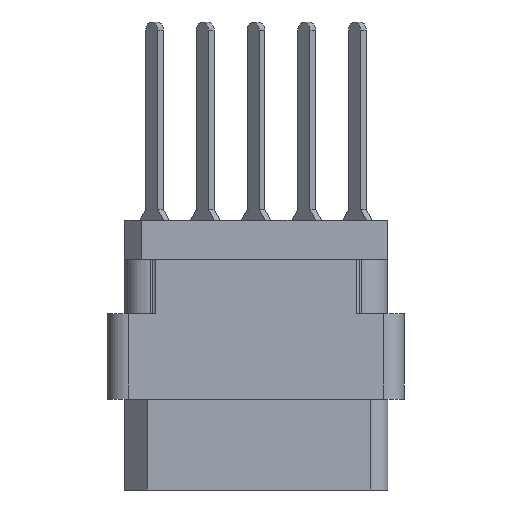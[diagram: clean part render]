
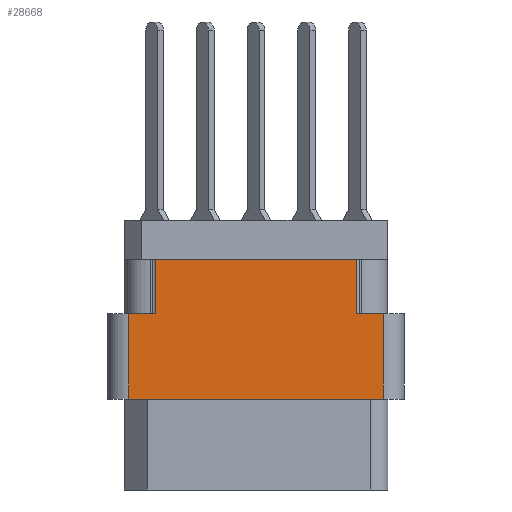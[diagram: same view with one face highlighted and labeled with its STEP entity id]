
A CAD part, left-side view. The second image highlights one B-rep face of the part: STEP entity #28668.
In plain terms, the highlighted planar face has unit normal (-1, 0, 0).
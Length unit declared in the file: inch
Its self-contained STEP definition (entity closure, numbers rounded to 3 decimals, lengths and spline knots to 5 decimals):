
#728 = CARTESIAN_POINT ( 'NONE',  ( -1., -0.376, -0.277 ) ) ;
#792 = LINE ( 'NONE', #17504, #22685 ) ;
#1238 = ORIENTED_EDGE ( 'NONE', *, *, #32346, .F. ) ;
#1358 = VECTOR ( 'NONE', #21945, 39.37008 ) ;
#1359 = EDGE_CURVE ( 'NONE', #29401, #2110, #792, .T. ) ;
#1814 = VECTOR ( 'NONE', #14646, 39.37008 ) ;
#2110 = VERTEX_POINT ( 'NONE', #22206 ) ;
#2185 = CARTESIAN_POINT ( 'NONE',  ( -1., -0.376, -0.529 ) ) ;
#2782 = CARTESIAN_POINT ( 'NONE',  ( -1., -0.376, -0.798 ) ) ;
#3081 = LINE ( 'NONE', #23075, #1814 ) ;
#3277 = DIRECTION ( 'NONE',  ( 0., -1., 0. ) ) ;
#3283 = CARTESIAN_POINT ( 'NONE',  ( -1., 0.376, -0.529 ) ) ;
#3299 = LINE ( 'NONE', #28642, #33651 ) ;
#4093 = DIRECTION ( 'NONE',  ( 0., -1., 0. ) ) ;
#4185 = VERTEX_POINT ( 'NONE', #6062 ) ;
#4687 = VERTEX_POINT ( 'NONE', #3283 ) ;
#4744 = VERTEX_POINT ( 'NONE', #35424 ) ;
#6062 = CARTESIAN_POINT ( 'NONE',  ( -1., -0.376, -0.529 ) ) ;
#6302 = EDGE_CURVE ( 'NONE', #4185, #4687, #10773, .T. ) ;
#7839 = VERTEX_POINT ( 'NONE', #728 ) ;
#8402 = CARTESIAN_POINT ( 'NONE',  ( -1., 0.438, -0.277 ) ) ;
#9349 = CARTESIAN_POINT ( 'NONE',  ( -1., 0.296, -0.277 ) ) ;
#9473 = VERTEX_POINT ( 'NONE', #10988 ) ;
#9908 = EDGE_CURVE ( 'NONE', #4744, #2110, #19010, .T. ) ;
#10062 = ORIENTED_EDGE ( 'NONE', *, *, #17559, .T. ) ;
#10773 = LINE ( 'NONE', #2185, #28179 ) ;
#10988 = CARTESIAN_POINT ( 'NONE',  ( -1., 0.376, -0.277 ) ) ;
#12277 = ORIENTED_EDGE ( 'NONE', *, *, #29274, .F. ) ;
#13438 = DIRECTION ( 'NONE',  ( 0., 0., 1. ) ) ;
#13970 = EDGE_LOOP ( 'NONE', ( #18472, #18614, #10062, #1238, #22683, #14006, #21763, #12277 ) ) ;
#14006 = ORIENTED_EDGE ( 'NONE', *, *, #1359, .F. ) ;
#14646 = DIRECTION ( 'NONE',  ( 0., 0., 1. ) ) ;
#14798 = DIRECTION ( 'NONE',  ( 0., 0., 1. ) ) ;
#15118 = VECTOR ( 'NONE', #3277, 39.37008 ) ;
#17504 = CARTESIAN_POINT ( 'NONE',  ( -1., 0.438, -0.117 ) ) ;
#17559 = EDGE_CURVE ( 'NONE', #4185, #7839, #3299, .T. ) ;
#18472 = ORIENTED_EDGE ( 'NONE', *, *, #19358, .F. ) ;
#18614 = ORIENTED_EDGE ( 'NONE', *, *, #6302, .F. ) ;
#19010 = LINE ( 'NONE', #33187, #1358 ) ;
#19358 = EDGE_CURVE ( 'NONE', #4687, #9473, #34122, .T. ) ;
#19970 = LINE ( 'NONE', #31565, #28435 ) ;
#21763 = ORIENTED_EDGE ( 'NONE', *, *, #24199, .F. ) ;
#21869 = PLANE ( 'NONE',  #32111 ) ;
#21945 = DIRECTION ( 'NONE',  ( 0., 0., 1. ) ) ;
#22206 = CARTESIAN_POINT ( 'NONE',  ( -1., -0.296, -0.117 ) ) ;
#22683 = ORIENTED_EDGE ( 'NONE', *, *, #9908, .T. ) ;
#22685 = VECTOR ( 'NONE', #4093, 39.37008 ) ;
#23075 = CARTESIAN_POINT ( 'NONE',  ( -1., 0.296, -0.277 ) ) ;
#24199 = EDGE_CURVE ( 'NONE', #30177, #29401, #3081, .T. ) ;
#25002 = FACE_OUTER_BOUND ( 'NONE', #13970, .T. ) ;
#25105 = DIRECTION ( 'NONE',  ( 0., 1., 0. ) ) ;
#28179 = VECTOR ( 'NONE', #25105, 39.37008 ) ;
#28246 = LINE ( 'NONE', #8402, #15118 ) ;
#28435 = VECTOR ( 'NONE', #31190, 39.37008 ) ;
#28642 = CARTESIAN_POINT ( 'NONE',  ( -1., -0.376, -0.798 ) ) ;
#28668 = ADVANCED_FACE ( 'NONE', ( #25002 ), #21869, .T. ) ;
#29166 = CARTESIAN_POINT ( 'NONE',  ( -1., 0.296, -0.117 ) ) ;
#29274 = EDGE_CURVE ( 'NONE', #9473, #30177, #28246, .T. ) ;
#29401 = VERTEX_POINT ( 'NONE', #29166 ) ;
#30177 = VERTEX_POINT ( 'NONE', #9349 ) ;
#31014 = CARTESIAN_POINT ( 'NONE',  ( -1., 0.376, -0.798 ) ) ;
#31190 = DIRECTION ( 'NONE',  ( 0., -1., 0. ) ) ;
#31214 = DIRECTION ( 'NONE',  ( 0., 0., 1. ) ) ;
#31565 = CARTESIAN_POINT ( 'NONE',  ( -1., -0.296, -0.277 ) ) ;
#32111 = AXIS2_PLACEMENT_3D ( 'NONE', #2782, #33106, #13438 ) ;
#32346 = EDGE_CURVE ( 'NONE', #4744, #7839, #19970, .T. ) ;
#33106 = DIRECTION ( 'NONE',  ( -1., 0., 0. ) ) ;
#33187 = CARTESIAN_POINT ( 'NONE',  ( -1., -0.296, -0.277 ) ) ;
#33651 = VECTOR ( 'NONE', #31214, 39.37008 ) ;
#34122 = LINE ( 'NONE', #31014, #35540 ) ;
#35424 = CARTESIAN_POINT ( 'NONE',  ( -1., -0.296, -0.277 ) ) ;
#35540 = VECTOR ( 'NONE', #14798, 39.37008 ) ;
